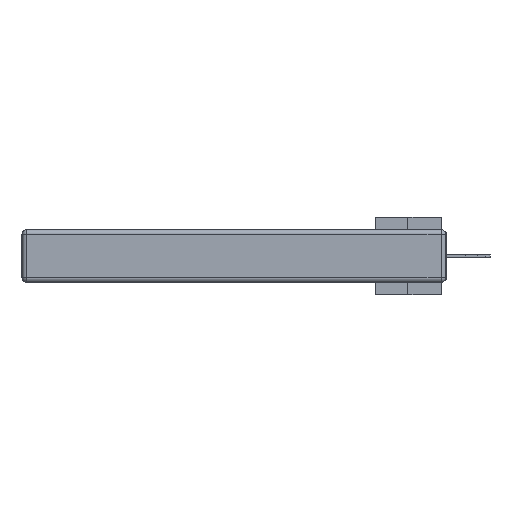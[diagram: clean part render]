
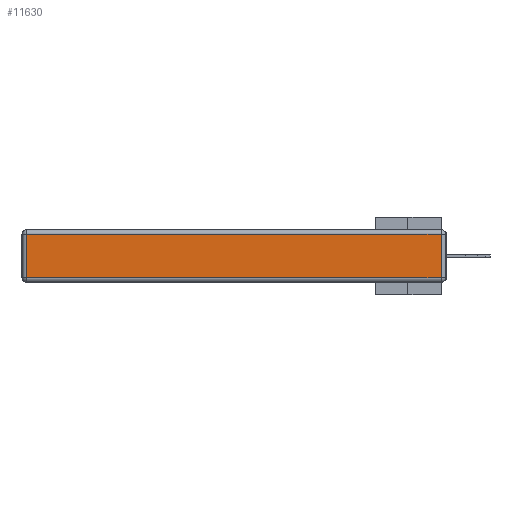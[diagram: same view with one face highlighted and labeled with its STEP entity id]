
A CAD part, left-side view. The second image highlights one B-rep face of the part: STEP entity #11630.
In plain terms, the highlighted planar face has unit normal (-1, 0, 0).
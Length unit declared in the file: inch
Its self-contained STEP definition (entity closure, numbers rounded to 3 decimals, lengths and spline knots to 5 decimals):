
#451 = VERTEX_POINT ( 'NONE', #16547 ) ;
#1072 = VECTOR ( 'NONE', #5906, 39.37008 ) ;
#1421 = EDGE_CURVE ( 'NONE', #15606, #451, #16837, .T. ) ;
#2619 = DIRECTION ( 'NONE',  ( 0., 0., 1. ) ) ;
#5906 = DIRECTION ( 'NONE',  ( 0., 0., -1. ) ) ;
#7085 = CARTESIAN_POINT ( 'NONE',  ( 0., 0.03, -0.343 ) ) ;
#7701 = CARTESIAN_POINT ( 'NONE',  ( 0., 0.03, -0.313 ) ) ;
#10179 = DIRECTION ( 'NONE',  ( 0., 0., 1. ) ) ;
#11228 = VERTEX_POINT ( 'NONE', #15270 ) ;
#11302 = CARTESIAN_POINT ( 'NONE',  ( 0., 0., -0.313 ) ) ;
#11630 = ADVANCED_FACE ( 'NONE', ( #17996 ), #36497, .T. ) ;
#11863 = LINE ( 'NONE', #36471, #24227 ) ;
#12200 = ORIENTED_EDGE ( 'NONE', *, *, #30962, .T. ) ;
#13225 = VERTEX_POINT ( 'NONE', #23040 ) ;
#14918 = VECTOR ( 'NONE', #10179, 39.37008 ) ;
#15217 = DIRECTION ( 'NONE',  ( 0., 1., 0. ) ) ;
#15270 = CARTESIAN_POINT ( 'NONE',  ( 0., 2.72, -0.313 ) ) ;
#15606 = VERTEX_POINT ( 'NONE', #7701 ) ;
#16547 = CARTESIAN_POINT ( 'NONE',  ( 0., 0.03, -0.03 ) ) ;
#16837 = LINE ( 'NONE', #7085, #14918 ) ;
#17029 = EDGE_CURVE ( 'NONE', #13225, #11228, #25489, .T. ) ;
#17159 = VECTOR ( 'NONE', #26488, 39.37008 ) ;
#17776 = CARTESIAN_POINT ( 'NONE',  ( 0., 0., -0.343 ) ) ;
#17996 = FACE_OUTER_BOUND ( 'NONE', #37936, .T. ) ;
#19564 = EDGE_CURVE ( 'NONE', #11228, #15606, #25261, .T. ) ;
#21951 = AXIS2_PLACEMENT_3D ( 'NONE', #17776, #27077, #2619 ) ;
#22484 = ORIENTED_EDGE ( 'NONE', *, *, #17029, .T. ) ;
#23040 = CARTESIAN_POINT ( 'NONE',  ( 0., 2.72, -0.03 ) ) ;
#24201 = CARTESIAN_POINT ( 'NONE',  ( 0., 2.72, -0.343 ) ) ;
#24227 = VECTOR ( 'NONE', #15217, 39.37008 ) ;
#25261 = LINE ( 'NONE', #11302, #17159 ) ;
#25489 = LINE ( 'NONE', #24201, #1072 ) ;
#26378 = ORIENTED_EDGE ( 'NONE', *, *, #19564, .T. ) ;
#26488 = DIRECTION ( 'NONE',  ( 0., -1., 0. ) ) ;
#27077 = DIRECTION ( 'NONE',  ( -1., 0., 0. ) ) ;
#30962 = EDGE_CURVE ( 'NONE', #451, #13225, #11863, .T. ) ;
#36471 = CARTESIAN_POINT ( 'NONE',  ( 0., 2.75, -0.03 ) ) ;
#36497 = PLANE ( 'NONE',  #21951 ) ;
#36772 = ORIENTED_EDGE ( 'NONE', *, *, #1421, .T. ) ;
#37936 = EDGE_LOOP ( 'NONE', ( #26378, #36772, #12200, #22484 ) ) ;
